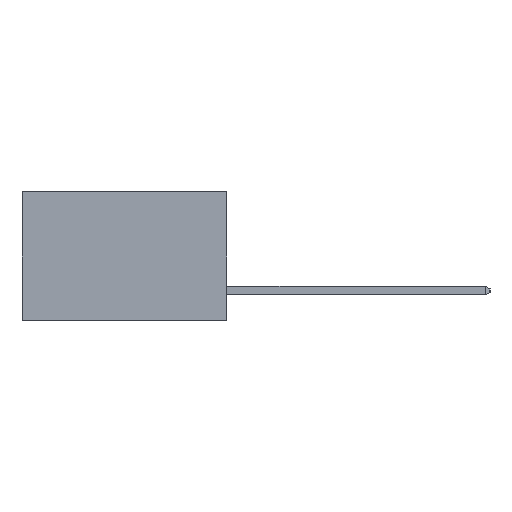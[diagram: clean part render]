
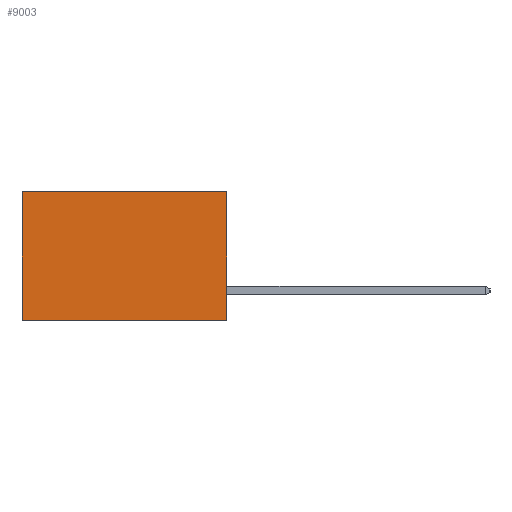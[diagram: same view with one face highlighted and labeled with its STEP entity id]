
A CAD part, left-side view. The second image highlights one B-rep face of the part: STEP entity #9003.
In plain terms, the highlighted planar face has unit normal (-1, 0, 0).
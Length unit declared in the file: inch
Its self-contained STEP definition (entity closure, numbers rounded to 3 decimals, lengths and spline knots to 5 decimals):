
#690 = DIRECTION ( 'NONE',  ( 0., 0., -1. ) ) ;
#797 = CARTESIAN_POINT ( 'NONE',  ( 0.277, 0.59, -0.37 ) ) ;
#868 = VECTOR ( 'NONE', #6984, 39.37008 ) ;
#1338 = CARTESIAN_POINT ( 'NONE',  ( 0.277, 0.59, -0.37 ) ) ;
#1401 = CARTESIAN_POINT ( 'NONE',  ( 0.277, 0., 0. ) ) ;
#2229 = VECTOR ( 'NONE', #690, 39.37008 ) ;
#2972 = CARTESIAN_POINT ( 'NONE',  ( 0.277, 0., -0.37 ) ) ;
#3191 = VECTOR ( 'NONE', #4327, 39.37008 ) ;
#3271 = ORIENTED_EDGE ( 'NONE', *, *, #7025, .F. ) ;
#3481 = LINE ( 'NONE', #7183, #868 ) ;
#3532 = PLANE ( 'NONE',  #6151 ) ;
#3580 = VERTEX_POINT ( 'NONE', #5701 ) ;
#3615 = ORIENTED_EDGE ( 'NONE', *, *, #7289, .F. ) ;
#4327 = DIRECTION ( 'NONE',  ( 0., 1., 0. ) ) ;
#4344 = VERTEX_POINT ( 'NONE', #1338 ) ;
#5291 = VECTOR ( 'NONE', #5466, 39.37008 ) ;
#5363 = CARTESIAN_POINT ( 'NONE',  ( 0.277, 0., -0.37 ) ) ;
#5466 = DIRECTION ( 'NONE',  ( 0., 0., -1. ) ) ;
#5622 = VERTEX_POINT ( 'NONE', #11031 ) ;
#5701 = CARTESIAN_POINT ( 'NONE',  ( 0.277, 0.59, 0. ) ) ;
#5763 = LINE ( 'NONE', #1401, #3191 ) ;
#6151 = AXIS2_PLACEMENT_3D ( 'NONE', #7323, #11785, #6419 ) ;
#6224 = EDGE_LOOP ( 'NONE', ( #11613, #3271, #3615, #7560 ) ) ;
#6419 = DIRECTION ( 'NONE',  ( 0., 0., -1. ) ) ;
#6984 = DIRECTION ( 'NONE',  ( 0., 1., 0. ) ) ;
#7025 = EDGE_CURVE ( 'NONE', #8622, #4344, #3481, .T. ) ;
#7183 = CARTESIAN_POINT ( 'NONE',  ( 0.277, 0., -0.37 ) ) ;
#7289 = EDGE_CURVE ( 'NONE', #5622, #8622, #7788, .T. ) ;
#7323 = CARTESIAN_POINT ( 'NONE',  ( 0.277, 0., -0.37 ) ) ;
#7324 = LINE ( 'NONE', #797, #2229 ) ;
#7560 = ORIENTED_EDGE ( 'NONE', *, *, #11310, .T. ) ;
#7733 = FACE_OUTER_BOUND ( 'NONE', #6224, .T. ) ;
#7788 = LINE ( 'NONE', #5363, #5291 ) ;
#8011 = EDGE_CURVE ( 'NONE', #3580, #4344, #7324, .T. ) ;
#8622 = VERTEX_POINT ( 'NONE', #2972 ) ;
#9003 = ADVANCED_FACE ( 'NONE', ( #7733 ), #3532, .F. ) ;
#11031 = CARTESIAN_POINT ( 'NONE',  ( 0.277, 0., 0. ) ) ;
#11310 = EDGE_CURVE ( 'NONE', #5622, #3580, #5763, .T. ) ;
#11613 = ORIENTED_EDGE ( 'NONE', *, *, #8011, .T. ) ;
#11785 = DIRECTION ( 'NONE',  ( 1., 0., 0. ) ) ;
